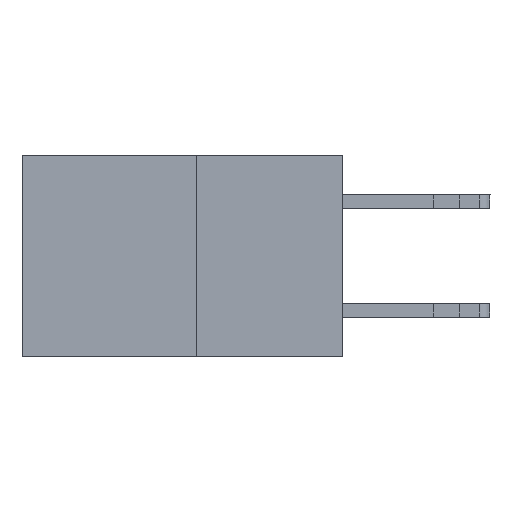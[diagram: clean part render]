
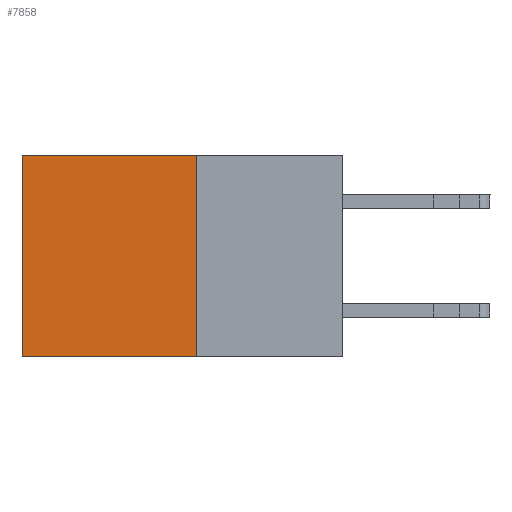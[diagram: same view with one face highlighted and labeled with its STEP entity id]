
A CAD part, left-side view. The second image highlights one B-rep face of the part: STEP entity #7858.
In plain terms, the highlighted planar face has unit normal (-1, 0, 0).
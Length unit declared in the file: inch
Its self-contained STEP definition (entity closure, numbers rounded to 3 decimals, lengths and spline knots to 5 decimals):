
#341 = EDGE_LOOP ( 'NONE', ( #4043, #9762, #6004, #10283 ) ) ;
#747 = FACE_OUTER_BOUND ( 'NONE', #341, .T. ) ;
#797 = LINE ( 'NONE', #3069, #9777 ) ;
#805 = DIRECTION ( 'NONE',  ( 0., 0., -1. ) ) ;
#1585 = AXIS2_PLACEMENT_3D ( 'NONE', #2472, #3153, #8217 ) ;
#2472 = CARTESIAN_POINT ( 'NONE',  ( 0.277, 0.27, -0.37 ) ) ;
#2517 = EDGE_CURVE ( 'NONE', #2617, #6591, #797, .T. ) ;
#2617 = VERTEX_POINT ( 'NONE', #8655 ) ;
#2618 = EDGE_CURVE ( 'NONE', #13023, #13615, #7037, .T. ) ;
#3069 = CARTESIAN_POINT ( 'NONE',  ( 0.277, 0.27, -0.37 ) ) ;
#3153 = DIRECTION ( 'NONE',  ( 1., 0., 0. ) ) ;
#3395 = EDGE_CURVE ( 'NONE', #13023, #2617, #8940, .T. ) ;
#3670 = CARTESIAN_POINT ( 'NONE',  ( 0.277, 0.59, -0.37 ) ) ;
#4000 = CARTESIAN_POINT ( 'NONE',  ( 0.277, 0.59, -0.37 ) ) ;
#4043 = ORIENTED_EDGE ( 'NONE', *, *, #8026, .T. ) ;
#4065 = VECTOR ( 'NONE', #12987, 39.37008 ) ;
#6004 = ORIENTED_EDGE ( 'NONE', *, *, #3395, .F. ) ;
#6557 = CARTESIAN_POINT ( 'NONE',  ( 0.277, 0.27, 0. ) ) ;
#6591 = VERTEX_POINT ( 'NONE', #4000 ) ;
#6747 = DIRECTION ( 'NONE',  ( 0., 1., 0. ) ) ;
#7037 = LINE ( 'NONE', #6557, #4065 ) ;
#7858 = ADVANCED_FACE ( 'NONE', ( #747 ), #9734, .F. ) ;
#7966 = CARTESIAN_POINT ( 'NONE',  ( 0.277, 0.27, 0. ) ) ;
#8026 = EDGE_CURVE ( 'NONE', #13615, #6591, #10232, .T. ) ;
#8217 = DIRECTION ( 'NONE',  ( 0., 0., -1. ) ) ;
#8648 = DIRECTION ( 'NONE',  ( 0., 0., -1. ) ) ;
#8655 = CARTESIAN_POINT ( 'NONE',  ( 0.277, 0.27, -0.37 ) ) ;
#8940 = LINE ( 'NONE', #12544, #11461 ) ;
#9734 = PLANE ( 'NONE',  #1585 ) ;
#9762 = ORIENTED_EDGE ( 'NONE', *, *, #2517, .F. ) ;
#9777 = VECTOR ( 'NONE', #6747, 39.37008 ) ;
#10232 = LINE ( 'NONE', #3670, #12790 ) ;
#10283 = ORIENTED_EDGE ( 'NONE', *, *, #2618, .T. ) ;
#11461 = VECTOR ( 'NONE', #805, 39.37008 ) ;
#12544 = CARTESIAN_POINT ( 'NONE',  ( 0.277, 0.27, -0.37 ) ) ;
#12790 = VECTOR ( 'NONE', #8648, 39.37008 ) ;
#12987 = DIRECTION ( 'NONE',  ( 0., 1., 0. ) ) ;
#13023 = VERTEX_POINT ( 'NONE', #7966 ) ;
#13281 = CARTESIAN_POINT ( 'NONE',  ( 0.277, 0.59, 0. ) ) ;
#13615 = VERTEX_POINT ( 'NONE', #13281 ) ;
